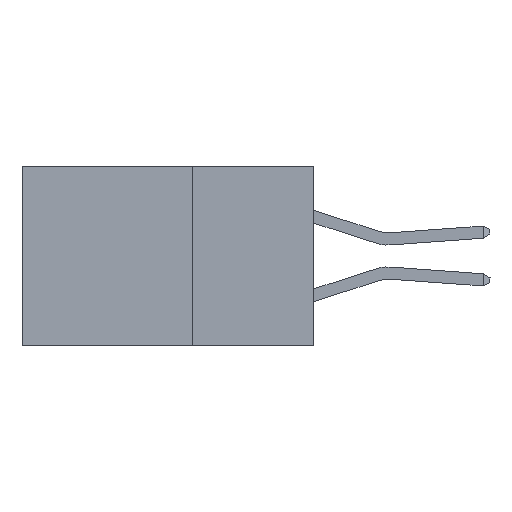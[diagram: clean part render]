
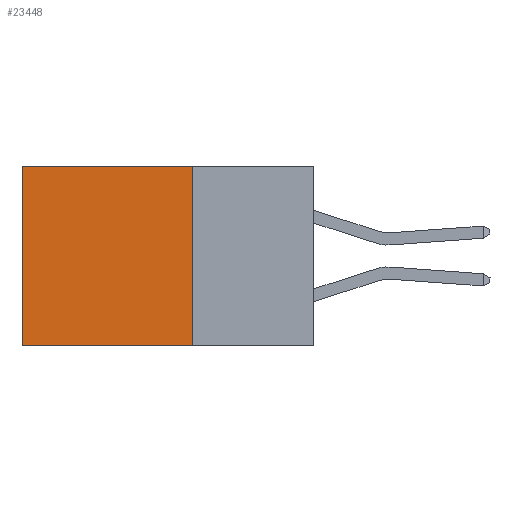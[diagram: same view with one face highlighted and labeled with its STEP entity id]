
A CAD part, left-side view. The second image highlights one B-rep face of the part: STEP entity #23448.
In plain terms, the highlighted planar face has unit normal (-1, 0, 0).
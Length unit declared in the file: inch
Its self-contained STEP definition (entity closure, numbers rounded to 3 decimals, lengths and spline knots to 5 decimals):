
#77 = CARTESIAN_POINT ( 'NONE',  ( 0.2875, 0.6, 0. ) ) ;
#1528 = ORIENTED_EDGE ( 'NONE', *, *, #28822, .T. ) ;
#2032 = FACE_OUTER_BOUND ( 'NONE', #24500, .T. ) ;
#2364 = VECTOR ( 'NONE', #7551, 39.37008 ) ;
#2570 = ORIENTED_EDGE ( 'NONE', *, *, #21871, .F. ) ;
#3294 = VERTEX_POINT ( 'NONE', #16234 ) ;
#4098 = VERTEX_POINT ( 'NONE', #8023 ) ;
#4174 = LINE ( 'NONE', #19030, #2364 ) ;
#4191 = DIRECTION ( 'NONE',  ( 0., 0., -1. ) ) ;
#6590 = CARTESIAN_POINT ( 'NONE',  ( 0.2875, 0.25, 0. ) ) ;
#7551 = DIRECTION ( 'NONE',  ( 0., 1., 0. ) ) ;
#7714 = CARTESIAN_POINT ( 'NONE',  ( 0.2875, 0.25, 0. ) ) ;
#7799 = DIRECTION ( 'NONE',  ( 0., 0., -1. ) ) ;
#8023 = CARTESIAN_POINT ( 'NONE',  ( 0.2875, 0.6, 0. ) ) ;
#8496 = CARTESIAN_POINT ( 'NONE',  ( 0.2875, 0.25, 0. ) ) ;
#9774 = ORIENTED_EDGE ( 'NONE', *, *, #21254, .T. ) ;
#11347 = VECTOR ( 'NONE', #15237, 39.37008 ) ;
#15237 = DIRECTION ( 'NONE',  ( 0., 1., 0. ) ) ;
#15357 = VECTOR ( 'NONE', #18825, 39.37008 ) ;
#16234 = CARTESIAN_POINT ( 'NONE',  ( 0.2875, 0.6, -0.37 ) ) ;
#16621 = VECTOR ( 'NONE', #4191, 39.37008 ) ;
#16804 = PLANE ( 'NONE',  #20127 ) ;
#17695 = LINE ( 'NONE', #6590, #16621 ) ;
#18825 = DIRECTION ( 'NONE',  ( 0., 0., -1. ) ) ;
#19030 = CARTESIAN_POINT ( 'NONE',  ( 0.2875, 0.25, 0. ) ) ;
#20127 = AXIS2_PLACEMENT_3D ( 'NONE', #7714, #25985, #7799 ) ;
#21254 = EDGE_CURVE ( 'NONE', #4098, #3294, #28934, .T. ) ;
#21871 = EDGE_CURVE ( 'NONE', #28242, #3294, #25639, .T. ) ;
#22298 = CARTESIAN_POINT ( 'NONE',  ( 0.2875, 0.25, -0.37 ) ) ;
#23448 = ADVANCED_FACE ( 'NONE', ( #2032 ), #16804, .F. ) ;
#23794 = EDGE_CURVE ( 'NONE', #25866, #28242, #17695, .T. ) ;
#24500 = EDGE_LOOP ( 'NONE', ( #9774, #2570, #27729, #1528 ) ) ;
#25550 = CARTESIAN_POINT ( 'NONE',  ( 0.2875, 0.25, -0.37 ) ) ;
#25639 = LINE ( 'NONE', #22298, #11347 ) ;
#25866 = VERTEX_POINT ( 'NONE', #8496 ) ;
#25985 = DIRECTION ( 'NONE',  ( 1., 0., 0. ) ) ;
#27729 = ORIENTED_EDGE ( 'NONE', *, *, #23794, .F. ) ;
#28242 = VERTEX_POINT ( 'NONE', #25550 ) ;
#28822 = EDGE_CURVE ( 'NONE', #25866, #4098, #4174, .T. ) ;
#28934 = LINE ( 'NONE', #77, #15357 ) ;
